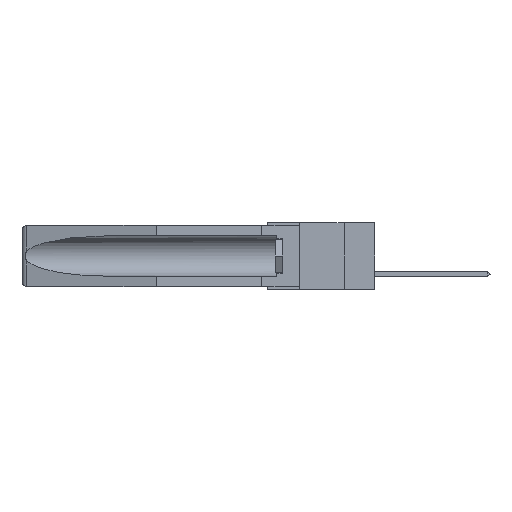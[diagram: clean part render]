
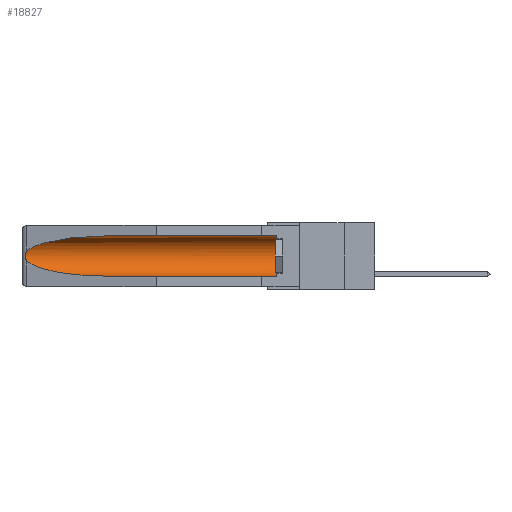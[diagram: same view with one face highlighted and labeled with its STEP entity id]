
A CAD part, left-side view. The second image highlights one B-rep face of the part: STEP entity #18827.
In plain terms, the highlighted cylindrical face has radius 2.857 mm (diameter 5.715 mm), a partial arc.
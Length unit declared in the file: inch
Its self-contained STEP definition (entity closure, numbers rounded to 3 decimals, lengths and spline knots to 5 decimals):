
#373 = CARTESIAN_POINT ( 'NONE',  ( 0.155, 0.126, -0.1715 ) ) ;
#594 = ORIENTED_EDGE ( 'NONE', *, *, #22313, .T. ) ;
#1143 = CARTESIAN_POINT ( 'NONE',  ( 0.155, 1.07973, -0.059 ) ) ;
#1163 = CARTESIAN_POINT ( 'NONE',  ( 0.26537, 1.52718, -0.19328 ) ) ;
#1576 = CARTESIAN_POINT ( 'NONE',  ( 0.21114, 1.30732, -0.284 ) ) ;
#2902 = CARTESIAN_POINT ( 'NONE',  ( 0.26537, 1.52718, -0.14972 ) ) ;
#2984 = B_SPLINE_CURVE_WITH_KNOTS ( 'NONE', 3,
 ( #5023, #14603, #18581, #18492, #6999, #6642, #16454, #20630, #20457, #1163 ),
 .UNSPECIFIED., .F., .F.,
 ( 4, 2, 2, 2, 4 ),
 ( 0., 0.00029, 0.00058, 0.00087, 0.00117 ),
 .UNSPECIFIED. ) ;
#3914 = ORIENTED_EDGE ( 'NONE', *, *, #4399, .F. ) ;
#4399 = EDGE_CURVE ( 'NONE', #21416, #6638, #22288, .T. ) ;
#5023 = CARTESIAN_POINT ( 'NONE',  ( 0.26537, 1.52718, -0.14972 ) ) ;
#5531 = AXIS2_PLACEMENT_3D ( 'NONE', #9179, #17011, #24579 ) ;
#5762 = VERTEX_POINT ( 'NONE', #22258 ) ;
#6288 = EDGE_CURVE ( 'NONE', #8545, #19154, #13918, .T. ) ;
#6368 = AXIS2_PLACEMENT_3D ( 'NONE', #373, #15615, #23417 ) ;
#6638 = VERTEX_POINT ( 'NONE', #8900 ) ;
#6642 = CARTESIAN_POINT ( 'NONE',  ( 0.2675, 1.53308, -0.17534 ) ) ;
#6999 = CARTESIAN_POINT ( 'NONE',  ( 0.2675, 1.53308, -0.16763 ) ) ;
#7879 = CARTESIAN_POINT ( 'NONE',  ( 0.26537, 1.52718, -0.14972 ) ) ;
#7973 = VECTOR ( 'NONE', #13182, 39.37008 ) ;
#8379 = ORIENTED_EDGE ( 'NONE', *, *, #6288, .T. ) ;
#8536 = EDGE_CURVE ( 'NONE', #10521, #8545, #15124, .T. ) ;
#8545 = VERTEX_POINT ( 'NONE', #10923 ) ;
#8815 = CARTESIAN_POINT ( 'NONE',  ( 0.155, 0.126, -0.059 ) ) ;
#8900 = CARTESIAN_POINT ( 'NONE',  ( 0.155, 1.07973, -0.284 ) ) ;
#9179 = CARTESIAN_POINT ( 'NONE',  ( 0.155, -0.30754, -0.1715 ) ) ;
#9299 = CARTESIAN_POINT ( 'NONE',  ( 0.26537, 1.52718, -0.19328 ) ) ;
#9382 = ORIENTED_EDGE ( 'NONE', *, *, #8536, .T. ) ;
#9802 = ORIENTED_EDGE ( 'NONE', *, *, #13835, .T. ) ;
#10521 = VERTEX_POINT ( 'NONE', #8815 ) ;
#10923 = CARTESIAN_POINT ( 'NONE',  ( 0.155, 1.07973, -0.059 ) ) ;
#11265 = CARTESIAN_POINT ( 'NONE',  ( 0.155, 1.07973, -0.284 ) ) ;
#11587 = CARTESIAN_POINT ( 'NONE',  ( 0.25451, 1.48313, -0.24835 ) ) ;
#11686 = EDGE_CURVE ( 'NONE', #19154, #5762, #2984, .T. ) ;
#11734 = VECTOR ( 'NONE', #22325, 39.37008 ) ;
#12529 = CARTESIAN_POINT ( 'NONE',  ( 0.25451, 1.48313, -0.09465 ) ) ;
#12539 = CARTESIAN_POINT ( 'NONE',  ( 0.155, -0.30754, -0.059 ) ) ;
#13160 =( BOUNDED_CURVE ( )  B_SPLINE_CURVE ( 3, ( #9299, #11587, #1576, #11265 ),
 .UNSPECIFIED., .F., .T. ) 
 B_SPLINE_CURVE_WITH_KNOTS ( ( 4, 4 ),
 ( 0.1948, 1.5708 ),
 .UNSPECIFIED. ) 
 CURVE ( )  GEOMETRIC_REPRESENTATION_ITEM ( )  RATIONAL_B_SPLINE_CURVE ( ( 1., 0.848, 0.848, 1. ) ) 
 REPRESENTATION_ITEM ( '' )  );
#13182 = DIRECTION ( 'NONE',  ( 0., 1., 0. ) ) ;
#13408 = CIRCLE ( 'NONE', #6368, 0.1125 ) ;
#13835 = EDGE_CURVE ( 'NONE', #5762, #6638, #13160, .T. ) ;
#13918 =( BOUNDED_CURVE ( )  B_SPLINE_CURVE ( 3, ( #1143, #22229, #12529, #2902 ),
 .UNSPECIFIED., .F., .T. ) 
 B_SPLINE_CURVE_WITH_KNOTS ( ( 4, 4 ),
 ( 4.71239, 6.08839 ),
 .UNSPECIFIED. ) 
 CURVE ( )  GEOMETRIC_REPRESENTATION_ITEM ( )  RATIONAL_B_SPLINE_CURVE ( ( 1., 0.848, 0.848, 1. ) ) 
 REPRESENTATION_ITEM ( '' )  );
#14552 = CARTESIAN_POINT ( 'NONE',  ( 0.155, 0.126, -0.284 ) ) ;
#14603 = CARTESIAN_POINT ( 'NONE',  ( 0.26597, 1.52961, -0.15275 ) ) ;
#15124 = LINE ( 'NONE', #12539, #11734 ) ;
#15615 = DIRECTION ( 'NONE',  ( 0., -1., 0. ) ) ;
#15827 = EDGE_LOOP ( 'NONE', ( #8379, #18094, #9802, #3914, #594, #9382 ) ) ;
#16454 = CARTESIAN_POINT ( 'NONE',  ( 0.2673, 1.53269, -0.17917 ) ) ;
#17011 = DIRECTION ( 'NONE',  ( 0., 1., 0. ) ) ;
#18094 = ORIENTED_EDGE ( 'NONE', *, *, #11686, .T. ) ;
#18492 = CARTESIAN_POINT ( 'NONE',  ( 0.2673, 1.5327, -0.16383 ) ) ;
#18581 = CARTESIAN_POINT ( 'NONE',  ( 0.26654, 1.53092, -0.15636 ) ) ;
#18827 = ADVANCED_FACE ( 'NONE', ( #22188 ), #21284, .F. ) ;
#19154 = VERTEX_POINT ( 'NONE', #7879 ) ;
#20457 = CARTESIAN_POINT ( 'NONE',  ( 0.26597, 1.5296, -0.19026 ) ) ;
#20630 = CARTESIAN_POINT ( 'NONE',  ( 0.26655, 1.53094, -0.18657 ) ) ;
#21284 = CYLINDRICAL_SURFACE ( 'NONE', #5531, 0.1125 ) ;
#21416 = VERTEX_POINT ( 'NONE', #14552 ) ;
#22188 = FACE_OUTER_BOUND ( 'NONE', #15827, .T. ) ;
#22229 = CARTESIAN_POINT ( 'NONE',  ( 0.21114, 1.30732, -0.059 ) ) ;
#22258 = CARTESIAN_POINT ( 'NONE',  ( 0.26537, 1.52718, -0.19328 ) ) ;
#22288 = LINE ( 'NONE', #24733, #7973 ) ;
#22313 = EDGE_CURVE ( 'NONE', #21416, #10521, #13408, .T. ) ;
#22325 = DIRECTION ( 'NONE',  ( 0., 1., 0. ) ) ;
#23417 = DIRECTION ( 'NONE',  ( 0., 0., 1. ) ) ;
#24579 = DIRECTION ( 'NONE',  ( 0., 0., 1. ) ) ;
#24733 = CARTESIAN_POINT ( 'NONE',  ( 0.155, -0.30754, -0.284 ) ) ;
